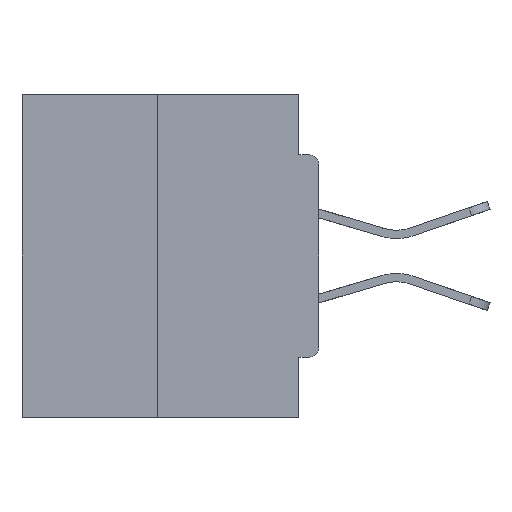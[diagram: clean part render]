
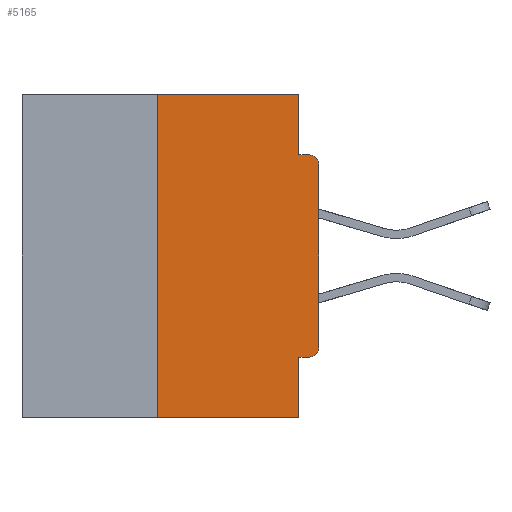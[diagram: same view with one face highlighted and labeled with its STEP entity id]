
A CAD part, left-side view. The second image highlights one B-rep face of the part: STEP entity #5165.
In plain terms, the highlighted planar face has unit normal (-1, 0, 0).
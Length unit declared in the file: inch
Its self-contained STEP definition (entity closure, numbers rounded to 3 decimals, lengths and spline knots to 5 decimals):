
#10 = LINE ( 'NONE', #27772, #21502 ) ;
#242 = DIRECTION ( 'NONE',  ( -1., 0., 0. ) ) ;
#579 = CARTESIAN_POINT ( 'NONE',  ( 0., 0., 0. ) ) ;
#1100 = PLANE ( 'NONE',  #20907 ) ;
#1339 = ORIENTED_EDGE ( 'NONE', *, *, #23914, .F. ) ;
#1464 = ORIENTED_EDGE ( 'NONE', *, *, #22749, .T. ) ;
#1511 = LINE ( 'NONE', #3615, #2328 ) ;
#1835 = EDGE_CURVE ( 'NONE', #1953, #26167, #19268, .T. ) ;
#1953 = VERTEX_POINT ( 'NONE', #16576 ) ;
#2328 = VECTOR ( 'NONE', #28611, 39.37008 ) ;
#2391 = EDGE_LOOP ( 'NONE', ( #31137, #1339, #6241, #4127, #19447, #12593, #3877, #1464, #26949, #19790 ) ) ;
#3615 = CARTESIAN_POINT ( 'NONE',  ( 0., 0.031, 0. ) ) ;
#3877 = ORIENTED_EDGE ( 'NONE', *, *, #1835, .T. ) ;
#4127 = ORIENTED_EDGE ( 'NONE', *, *, #22663, .F. ) ;
#4796 = VECTOR ( 'NONE', #12299, 39.37008 ) ;
#4840 = AXIS2_PLACEMENT_3D ( 'NONE', #22943, #242, #25425 ) ;
#5165 = ADVANCED_FACE ( 'NONE', ( #28671 ), #1100, .F. ) ;
#5376 = VECTOR ( 'NONE', #28526, 39.37008 ) ;
#6241 = ORIENTED_EDGE ( 'NONE', *, *, #16548, .T. ) ;
#6391 = VECTOR ( 'NONE', #11513, 39.37008 ) ;
#6684 = CARTESIAN_POINT ( 'NONE',  ( 0., 0.25, 0. ) ) ;
#6760 = CARTESIAN_POINT ( 'NONE',  ( 0., 0.015, -0.1085 ) ) ;
#7630 = EDGE_CURVE ( 'NONE', #9704, #25085, #20891, .T. ) ;
#7841 = CARTESIAN_POINT ( 'NONE',  ( 0., 0.031, -0.4065 ) ) ;
#8613 = DIRECTION ( 'NONE',  ( 0., 0., -1. ) ) ;
#8892 = CARTESIAN_POINT ( 'NONE',  ( 0., 0.25, -0.5 ) ) ;
#9156 = VECTOR ( 'NONE', #31441, 39.37008 ) ;
#9422 = DIRECTION ( 'NONE',  ( -1., 0., 0. ) ) ;
#9704 = VERTEX_POINT ( 'NONE', #6684 ) ;
#10545 = DIRECTION ( 'NONE',  ( 0., 0., 1. ) ) ;
#10788 = VERTEX_POINT ( 'NONE', #15091 ) ;
#11197 = EDGE_CURVE ( 'NONE', #28745, #20206, #29997, .T. ) ;
#11513 = DIRECTION ( 'NONE',  ( 0., 0., -1. ) ) ;
#12299 = DIRECTION ( 'NONE',  ( 0., -1., 0. ) ) ;
#12593 = ORIENTED_EDGE ( 'NONE', *, *, #18413, .T. ) ;
#15088 = VERTEX_POINT ( 'NONE', #17177 ) ;
#15091 = CARTESIAN_POINT ( 'NONE',  ( 0., 0.015, -0.0935 ) ) ;
#16460 = VECTOR ( 'NONE', #10545, 39.37008 ) ;
#16548 = EDGE_CURVE ( 'NONE', #19836, #31282, #25523, .T. ) ;
#16576 = CARTESIAN_POINT ( 'NONE',  ( 0., 0., -0.3915 ) ) ;
#16801 = DIRECTION ( 'NONE',  ( 1., 0., 0. ) ) ;
#16906 = VECTOR ( 'NONE', #24911, 39.37008 ) ;
#17177 = CARTESIAN_POINT ( 'NONE',  ( 0., 0.031, -0.0935 ) ) ;
#17181 = CIRCLE ( 'NONE', #23709, 0.015 ) ;
#18413 = EDGE_CURVE ( 'NONE', #28745, #1953, #26590, .T. ) ;
#19026 = CARTESIAN_POINT ( 'NONE',  ( 0., 0.46, 0. ) ) ;
#19268 = LINE ( 'NONE', #579, #16460 ) ;
#19447 = ORIENTED_EDGE ( 'NONE', *, *, #11197, .F. ) ;
#19770 = CARTESIAN_POINT ( 'NONE',  ( 0., 0.015, -0.4065 ) ) ;
#19790 = ORIENTED_EDGE ( 'NONE', *, *, #24359, .F. ) ;
#19836 = VERTEX_POINT ( 'NONE', #8892 ) ;
#20206 = VERTEX_POINT ( 'NONE', #7841 ) ;
#20891 = LINE ( 'NONE', #29747, #16906 ) ;
#20907 = AXIS2_PLACEMENT_3D ( 'NONE', #19026, #16801, #8613 ) ;
#21502 = VECTOR ( 'NONE', #27537, 39.37008 ) ;
#21781 = CARTESIAN_POINT ( 'NONE',  ( 0., 0., -0.4065 ) ) ;
#22663 = EDGE_CURVE ( 'NONE', #20206, #31282, #24773, .T. ) ;
#22749 = EDGE_CURVE ( 'NONE', #26167, #10788, #17181, .T. ) ;
#22943 = CARTESIAN_POINT ( 'NONE',  ( 0., 0.015, -0.3915 ) ) ;
#23204 = CARTESIAN_POINT ( 'NONE',  ( 0., 0.031, 0. ) ) ;
#23474 = CARTESIAN_POINT ( 'NONE',  ( 0., 0.031, -0.5 ) ) ;
#23709 = AXIS2_PLACEMENT_3D ( 'NONE', #6760, #9422, #27327 ) ;
#23914 = EDGE_CURVE ( 'NONE', #19836, #9704, #10, .T. ) ;
#24145 = CARTESIAN_POINT ( 'NONE',  ( 0., 0.031, -0.5 ) ) ;
#24359 = EDGE_CURVE ( 'NONE', #25085, #15088, #1511, .T. ) ;
#24773 = LINE ( 'NONE', #24145, #6391 ) ;
#24911 = DIRECTION ( 'NONE',  ( 0., -1., 0. ) ) ;
#25085 = VERTEX_POINT ( 'NONE', #23204 ) ;
#25188 = CARTESIAN_POINT ( 'NONE',  ( 0., 0., -0.0935 ) ) ;
#25425 = DIRECTION ( 'NONE',  ( 0., 0., -1. ) ) ;
#25523 = LINE ( 'NONE', #27970, #4796 ) ;
#25731 = EDGE_CURVE ( 'NONE', #15088, #10788, #31810, .T. ) ;
#26110 = CARTESIAN_POINT ( 'NONE',  ( 0., 0., -0.1085 ) ) ;
#26167 = VERTEX_POINT ( 'NONE', #26110 ) ;
#26590 = CIRCLE ( 'NONE', #4840, 0.015 ) ;
#26949 = ORIENTED_EDGE ( 'NONE', *, *, #25731, .F. ) ;
#27327 = DIRECTION ( 'NONE',  ( 0., 0., -1. ) ) ;
#27537 = DIRECTION ( 'NONE',  ( 0., 0., 1. ) ) ;
#27772 = CARTESIAN_POINT ( 'NONE',  ( 0., 0.25, 0. ) ) ;
#27970 = CARTESIAN_POINT ( 'NONE',  ( 0., 0.46, -0.5 ) ) ;
#28526 = DIRECTION ( 'NONE',  ( 0., -1., 0. ) ) ;
#28611 = DIRECTION ( 'NONE',  ( 0., 0., -1. ) ) ;
#28671 = FACE_OUTER_BOUND ( 'NONE', #2391, .T. ) ;
#28745 = VERTEX_POINT ( 'NONE', #19770 ) ;
#29747 = CARTESIAN_POINT ( 'NONE',  ( 0., 0.46, 0. ) ) ;
#29997 = LINE ( 'NONE', #21781, #9156 ) ;
#31137 = ORIENTED_EDGE ( 'NONE', *, *, #7630, .F. ) ;
#31282 = VERTEX_POINT ( 'NONE', #23474 ) ;
#31441 = DIRECTION ( 'NONE',  ( 0., 1., 0. ) ) ;
#31810 = LINE ( 'NONE', #25188, #5376 ) ;
